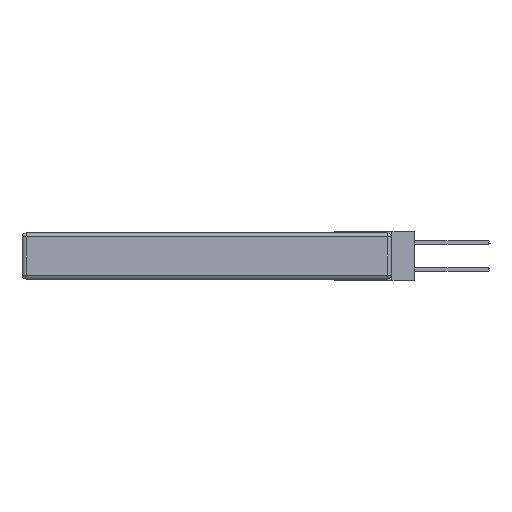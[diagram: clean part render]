
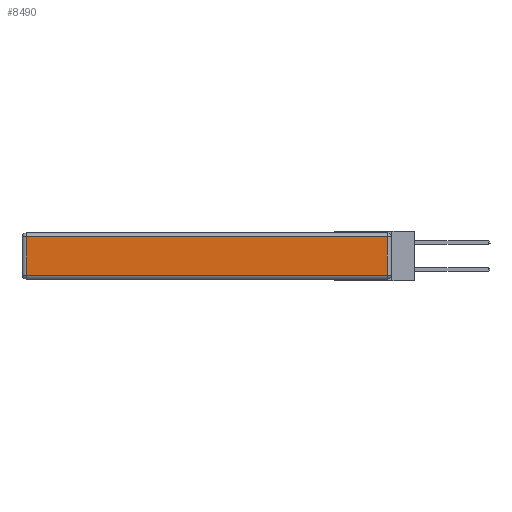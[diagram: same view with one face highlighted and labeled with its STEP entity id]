
A CAD part, left-side view. The second image highlights one B-rep face of the part: STEP entity #8490.
In plain terms, the highlighted planar face has unit normal (-1, 0, 0).
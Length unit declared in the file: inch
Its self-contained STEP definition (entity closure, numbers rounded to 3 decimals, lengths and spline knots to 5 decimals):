
#333 = EDGE_LOOP ( 'NONE', ( #3394, #9818, #6458, #1433 ) ) ;
#340 = VERTEX_POINT ( 'NONE', #425 ) ;
#425 = CARTESIAN_POINT ( 'NONE',  ( 0., 0.03, -0.03 ) ) ;
#472 = DIRECTION ( 'NONE',  ( -1., 0., 0. ) ) ;
#1001 = VERTEX_POINT ( 'NONE', #9661 ) ;
#1221 = CARTESIAN_POINT ( 'NONE',  ( 0., 2.72, -0.03 ) ) ;
#1433 = ORIENTED_EDGE ( 'NONE', *, *, #11017, .T. ) ;
#2296 = VECTOR ( 'NONE', #11650, 39.37008 ) ;
#2720 = LINE ( 'NONE', #8937, #6390 ) ;
#2827 = CARTESIAN_POINT ( 'NONE',  ( 0., 0., -0.343 ) ) ;
#3297 = CARTESIAN_POINT ( 'NONE',  ( 0., 2.72, -0.313 ) ) ;
#3394 = ORIENTED_EDGE ( 'NONE', *, *, #11037, .T. ) ;
#4749 = PLANE ( 'NONE',  #10760 ) ;
#5128 = EDGE_CURVE ( 'NONE', #340, #6660, #8628, .T. ) ;
#5144 = DIRECTION ( 'NONE',  ( 0., 0., -1. ) ) ;
#5399 = LINE ( 'NONE', #5934, #2296 ) ;
#5454 = CARTESIAN_POINT ( 'NONE',  ( 0., 2.75, -0.03 ) ) ;
#5934 = CARTESIAN_POINT ( 'NONE',  ( 0., 0., -0.313 ) ) ;
#6390 = VECTOR ( 'NONE', #6708, 39.37008 ) ;
#6458 = ORIENTED_EDGE ( 'NONE', *, *, #5128, .T. ) ;
#6660 = VERTEX_POINT ( 'NONE', #1221 ) ;
#6684 = EDGE_CURVE ( 'NONE', #1001, #340, #2720, .T. ) ;
#6708 = DIRECTION ( 'NONE',  ( 0., 0., 1. ) ) ;
#8426 = CARTESIAN_POINT ( 'NONE',  ( 0., 2.72, -0.343 ) ) ;
#8490 = ADVANCED_FACE ( 'NONE', ( #9100 ), #4749, .T. ) ;
#8628 = LINE ( 'NONE', #5454, #9812 ) ;
#8937 = CARTESIAN_POINT ( 'NONE',  ( 0., 0.03, -0.343 ) ) ;
#9100 = FACE_OUTER_BOUND ( 'NONE', #333, .T. ) ;
#9219 = DIRECTION ( 'NONE',  ( 0., 1., 0. ) ) ;
#9661 = CARTESIAN_POINT ( 'NONE',  ( 0., 0.03, -0.313 ) ) ;
#9707 = DIRECTION ( 'NONE',  ( 0., 0., 1. ) ) ;
#9812 = VECTOR ( 'NONE', #9219, 39.37008 ) ;
#9818 = ORIENTED_EDGE ( 'NONE', *, *, #6684, .T. ) ;
#10568 = LINE ( 'NONE', #8426, #12187 ) ;
#10760 = AXIS2_PLACEMENT_3D ( 'NONE', #2827, #472, #9707 ) ;
#11017 = EDGE_CURVE ( 'NONE', #6660, #11060, #10568, .T. ) ;
#11037 = EDGE_CURVE ( 'NONE', #11060, #1001, #5399, .T. ) ;
#11060 = VERTEX_POINT ( 'NONE', #3297 ) ;
#11650 = DIRECTION ( 'NONE',  ( 0., -1., 0. ) ) ;
#12187 = VECTOR ( 'NONE', #5144, 39.37008 ) ;
